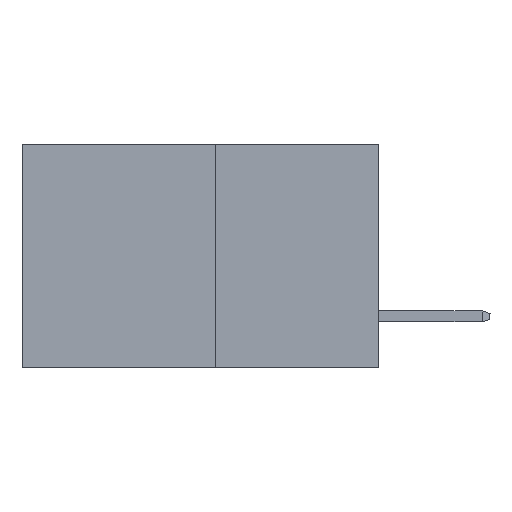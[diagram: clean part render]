
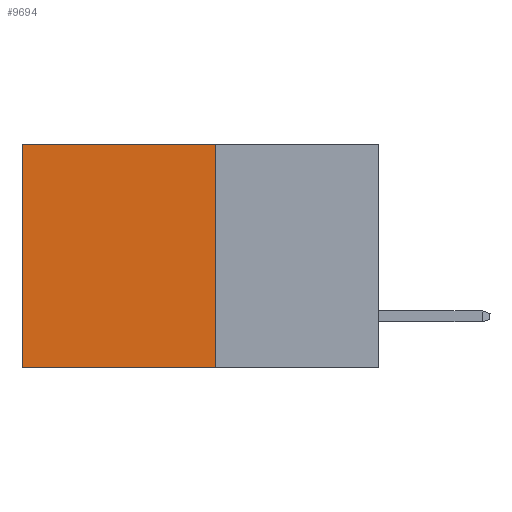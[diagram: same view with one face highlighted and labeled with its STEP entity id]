
A CAD part, left-side view. The second image highlights one B-rep face of the part: STEP entity #9694.
In plain terms, the highlighted planar face has unit normal (-1, 0, 0).
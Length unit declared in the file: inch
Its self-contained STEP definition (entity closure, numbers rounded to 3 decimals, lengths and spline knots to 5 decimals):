
#155 = VERTEX_POINT ( 'NONE', #5091 ) ;
#625 = LINE ( 'NONE', #18053, #11469 ) ;
#2387 = VECTOR ( 'NONE', #19915, 39.37008 ) ;
#2660 = CARTESIAN_POINT ( 'NONE',  ( 0.277, 0.27, -0.37 ) ) ;
#2812 = VECTOR ( 'NONE', #9379, 39.37008 ) ;
#2848 = PLANE ( 'NONE',  #8825 ) ;
#2891 = CARTESIAN_POINT ( 'NONE',  ( 0.277, 0.59, -0.37 ) ) ;
#3062 = LINE ( 'NONE', #2660, #2387 ) ;
#3376 = CARTESIAN_POINT ( 'NONE',  ( 0.277, 0.59, -0.37 ) ) ;
#5091 = CARTESIAN_POINT ( 'NONE',  ( 0.277, 0.27, 0. ) ) ;
#5556 = DIRECTION ( 'NONE',  ( 0., 0., -1. ) ) ;
#5898 = CARTESIAN_POINT ( 'NONE',  ( 0.277, 0.27, -0.37 ) ) ;
#6388 = EDGE_CURVE ( 'NONE', #155, #10089, #20665, .T. ) ;
#6931 = ORIENTED_EDGE ( 'NONE', *, *, #16221, .T. ) ;
#7199 = DIRECTION ( 'NONE',  ( 1., 0., 0. ) ) ;
#7433 = ORIENTED_EDGE ( 'NONE', *, *, #6388, .T. ) ;
#8825 = AXIS2_PLACEMENT_3D ( 'NONE', #9298, #7199, #22265 ) ;
#8920 = CARTESIAN_POINT ( 'NONE',  ( 0.277, 0.27, 0. ) ) ;
#9298 = CARTESIAN_POINT ( 'NONE',  ( 0.277, 0.27, -0.37 ) ) ;
#9379 = DIRECTION ( 'NONE',  ( 0., 1., 0. ) ) ;
#9694 = ADVANCED_FACE ( 'NONE', ( #18143 ), #2848, .F. ) ;
#10089 = VERTEX_POINT ( 'NONE', #24024 ) ;
#10887 = VERTEX_POINT ( 'NONE', #2891 ) ;
#11188 = VERTEX_POINT ( 'NONE', #5898 ) ;
#11469 = VECTOR ( 'NONE', #15890, 39.37008 ) ;
#11634 = EDGE_CURVE ( 'NONE', #155, #11188, #625, .T. ) ;
#12996 = ORIENTED_EDGE ( 'NONE', *, *, #24628, .F. ) ;
#14921 = LINE ( 'NONE', #3376, #25634 ) ;
#15890 = DIRECTION ( 'NONE',  ( 0., 0., -1. ) ) ;
#16221 = EDGE_CURVE ( 'NONE', #10089, #10887, #14921, .T. ) ;
#18053 = CARTESIAN_POINT ( 'NONE',  ( 0.277, 0.27, -0.37 ) ) ;
#18143 = FACE_OUTER_BOUND ( 'NONE', #27063, .T. ) ;
#19915 = DIRECTION ( 'NONE',  ( 0., 1., 0. ) ) ;
#20665 = LINE ( 'NONE', #8920, #2812 ) ;
#21006 = ORIENTED_EDGE ( 'NONE', *, *, #11634, .F. ) ;
#22265 = DIRECTION ( 'NONE',  ( 0., 0., -1. ) ) ;
#24024 = CARTESIAN_POINT ( 'NONE',  ( 0.277, 0.59, 0. ) ) ;
#24628 = EDGE_CURVE ( 'NONE', #11188, #10887, #3062, .T. ) ;
#25634 = VECTOR ( 'NONE', #5556, 39.37008 ) ;
#27063 = EDGE_LOOP ( 'NONE', ( #6931, #12996, #21006, #7433 ) ) ;
